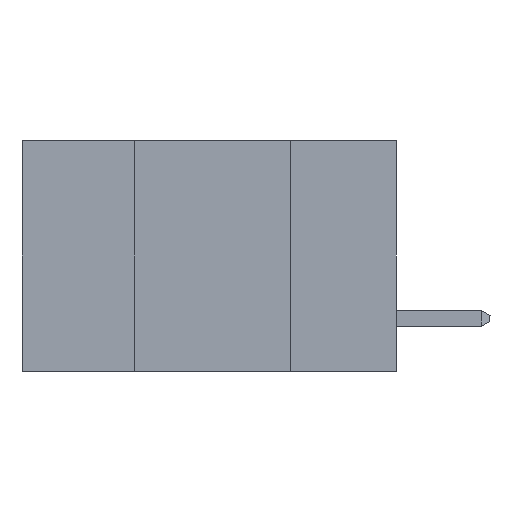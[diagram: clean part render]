
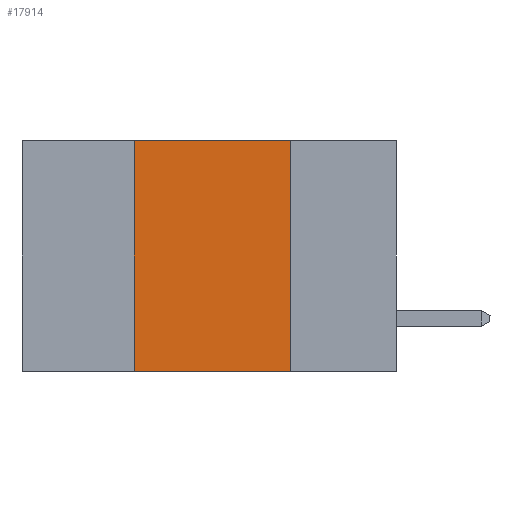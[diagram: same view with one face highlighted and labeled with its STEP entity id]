
A CAD part, left-side view. The second image highlights one B-rep face of the part: STEP entity #17914.
In plain terms, the highlighted planar face has unit normal (-1, 0, 0).
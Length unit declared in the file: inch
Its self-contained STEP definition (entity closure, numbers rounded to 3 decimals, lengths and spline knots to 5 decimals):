
#796 = EDGE_LOOP ( 'NONE', ( #2125, #2607, #7259, #12776 ) ) ;
#1619 = LINE ( 'NONE', #16275, #13746 ) ;
#1924 = VECTOR ( 'NONE', #19369, 39.37008 ) ;
#2125 = ORIENTED_EDGE ( 'NONE', *, *, #6777, .F. ) ;
#2436 = FACE_OUTER_BOUND ( 'NONE', #796, .T. ) ;
#2560 = EDGE_CURVE ( 'NONE', #5586, #19256, #9768, .T. ) ;
#2607 = ORIENTED_EDGE ( 'NONE', *, *, #5713, .F. ) ;
#3624 = EDGE_CURVE ( 'NONE', #5586, #9429, #1619, .T. ) ;
#3959 = DIRECTION ( 'NONE',  ( 0., 0., -1. ) ) ;
#4178 = CARTESIAN_POINT ( 'NONE',  ( 0., 0.17, -0.37 ) ) ;
#4353 = VECTOR ( 'NONE', #3959, 39.37008 ) ;
#4716 = DIRECTION ( 'NONE',  ( 0., -1., 0. ) ) ;
#4784 = CARTESIAN_POINT ( 'NONE',  ( 0., 0.6, 0. ) ) ;
#5586 = VERTEX_POINT ( 'NONE', #6876 ) ;
#5713 = EDGE_CURVE ( 'NONE', #9429, #8372, #15381, .T. ) ;
#6666 = PLANE ( 'NONE',  #11128 ) ;
#6777 = EDGE_CURVE ( 'NONE', #8372, #19256, #9508, .T. ) ;
#6876 = CARTESIAN_POINT ( 'NONE',  ( 0., 0.42, -0.37 ) ) ;
#7259 = ORIENTED_EDGE ( 'NONE', *, *, #3624, .F. ) ;
#7482 = CARTESIAN_POINT ( 'NONE',  ( 0., 0.17, 0. ) ) ;
#8226 = DIRECTION ( 'NONE',  ( 1., 0., 0. ) ) ;
#8372 = VERTEX_POINT ( 'NONE', #7482 ) ;
#9429 = VERTEX_POINT ( 'NONE', #12412 ) ;
#9508 = LINE ( 'NONE', #4178, #4353 ) ;
#9768 = LINE ( 'NONE', #19457, #1924 ) ;
#11128 = AXIS2_PLACEMENT_3D ( 'NONE', #17649, #8226, #19169 ) ;
#11144 = VECTOR ( 'NONE', #4716, 39.37008 ) ;
#12412 = CARTESIAN_POINT ( 'NONE',  ( 0., 0.42, 0. ) ) ;
#12776 = ORIENTED_EDGE ( 'NONE', *, *, #2560, .T. ) ;
#13746 = VECTOR ( 'NONE', #16098, 39.37008 ) ;
#15381 = LINE ( 'NONE', #4784, #11144 ) ;
#16098 = DIRECTION ( 'NONE',  ( 0., 0., 1. ) ) ;
#16275 = CARTESIAN_POINT ( 'NONE',  ( 0., 0.42, -0.37 ) ) ;
#17649 = CARTESIAN_POINT ( 'NONE',  ( 0., 0.6, 0. ) ) ;
#17914 = ADVANCED_FACE ( 'NONE', ( #2436 ), #6666, .F. ) ;
#19169 = DIRECTION ( 'NONE',  ( 0., 0., -1. ) ) ;
#19256 = VERTEX_POINT ( 'NONE', #20124 ) ;
#19369 = DIRECTION ( 'NONE',  ( 0., -1., 0. ) ) ;
#19457 = CARTESIAN_POINT ( 'NONE',  ( 0., 0.6, -0.37 ) ) ;
#20124 = CARTESIAN_POINT ( 'NONE',  ( 0., 0.17, -0.37 ) ) ;
